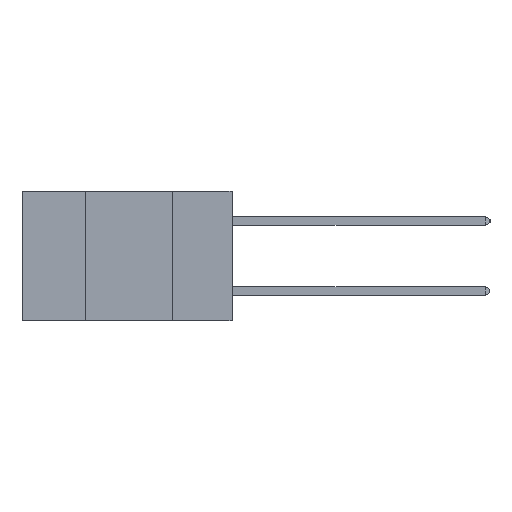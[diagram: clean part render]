
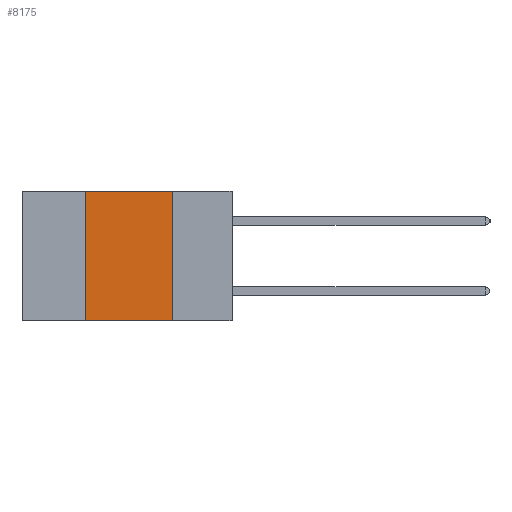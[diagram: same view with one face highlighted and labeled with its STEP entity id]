
A CAD part, left-side view. The second image highlights one B-rep face of the part: STEP entity #8175.
In plain terms, the highlighted planar face has unit normal (-1, 0, 0).
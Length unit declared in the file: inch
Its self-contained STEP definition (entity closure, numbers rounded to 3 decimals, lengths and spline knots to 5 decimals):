
#481 = ORIENTED_EDGE ( 'NONE', *, *, #1877, .F. ) ;
#1065 = VERTEX_POINT ( 'NONE', #5845 ) ;
#1257 = ORIENTED_EDGE ( 'NONE', *, *, #13429, .F. ) ;
#1266 = AXIS2_PLACEMENT_3D ( 'NONE', #9882, #11856, #5276 ) ;
#1877 = EDGE_CURVE ( 'NONE', #1065, #3281, #2718, .T. ) ;
#2718 = LINE ( 'NONE', #3372, #8573 ) ;
#2905 = VERTEX_POINT ( 'NONE', #5834 ) ;
#2912 = VERTEX_POINT ( 'NONE', #6139 ) ;
#3281 = VERTEX_POINT ( 'NONE', #5046 ) ;
#3342 = DIRECTION ( 'NONE',  ( 0., 0., -1. ) ) ;
#3372 = CARTESIAN_POINT ( 'NONE',  ( 0., 0.17, 0. ) ) ;
#3726 = ORIENTED_EDGE ( 'NONE', *, *, #6260, .F. ) ;
#3805 = LINE ( 'NONE', #6120, #13149 ) ;
#5046 = CARTESIAN_POINT ( 'NONE',  ( 0., 0.17, -0.37 ) ) ;
#5096 = LINE ( 'NONE', #12420, #7922 ) ;
#5276 = DIRECTION ( 'NONE',  ( 0., 0., -1. ) ) ;
#5834 = CARTESIAN_POINT ( 'NONE',  ( 0., 0.42, 0. ) ) ;
#5845 = CARTESIAN_POINT ( 'NONE',  ( 0., 0.17, 0. ) ) ;
#6103 = DIRECTION ( 'NONE',  ( 0., -1., 0. ) ) ;
#6120 = CARTESIAN_POINT ( 'NONE',  ( 0., 0.6, 0. ) ) ;
#6139 = CARTESIAN_POINT ( 'NONE',  ( 0., 0.42, -0.37 ) ) ;
#6260 = EDGE_CURVE ( 'NONE', #2905, #1065, #3805, .T. ) ;
#6542 = EDGE_LOOP ( 'NONE', ( #481, #3726, #1257, #8782 ) ) ;
#7922 = VECTOR ( 'NONE', #13406, 39.37008 ) ;
#8175 = ADVANCED_FACE ( 'NONE', ( #10535 ), #10839, .F. ) ;
#8573 = VECTOR ( 'NONE', #3342, 39.37008 ) ;
#8782 = ORIENTED_EDGE ( 'NONE', *, *, #12772, .T. ) ;
#9487 = LINE ( 'NONE', #11225, #11801 ) ;
#9882 = CARTESIAN_POINT ( 'NONE',  ( 0., 0.6, 0. ) ) ;
#10535 = FACE_OUTER_BOUND ( 'NONE', #6542, .T. ) ;
#10839 = PLANE ( 'NONE',  #1266 ) ;
#11225 = CARTESIAN_POINT ( 'NONE',  ( 0., 0.42, 0. ) ) ;
#11801 = VECTOR ( 'NONE', #12185, 39.37008 ) ;
#11856 = DIRECTION ( 'NONE',  ( 1., 0., 0. ) ) ;
#12185 = DIRECTION ( 'NONE',  ( 0., 0., 1. ) ) ;
#12420 = CARTESIAN_POINT ( 'NONE',  ( 0., 0.6, -0.37 ) ) ;
#12772 = EDGE_CURVE ( 'NONE', #2912, #3281, #5096, .T. ) ;
#13149 = VECTOR ( 'NONE', #6103, 39.37008 ) ;
#13406 = DIRECTION ( 'NONE',  ( 0., -1., 0. ) ) ;
#13429 = EDGE_CURVE ( 'NONE', #2912, #2905, #9487, .T. ) ;
